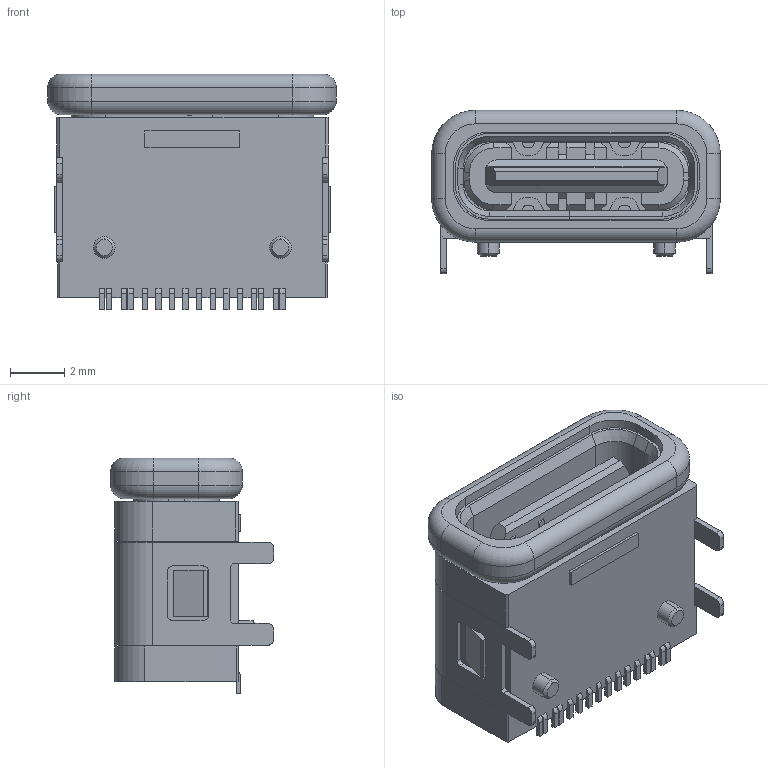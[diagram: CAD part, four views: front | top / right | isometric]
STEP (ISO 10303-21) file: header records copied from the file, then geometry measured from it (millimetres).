
FILE_DESCRIPTION (( 'STEP AP214' ), '1' );
FILE_NAME ('698B116W163-601.STEP', '2021-01-15T13:41:08', ( '' ), ( '' ), 'SwSTEP 2.0', 'SolidWorks 2020', '' );
FILE_SCHEMA (( 'AUTOMOTIVE_DESIGN' ));
Length unit declared in the file: millimetre
Products named in the file (5): Shell1 698B116WX63-601; 698B116WX63-601 (Seal); Shell2 698B116WX63-601; 698B116W163-601; Insulator 698B116WX63-601
Assembly tree (4 placements, depth 2):
  698B116W163-601
    Insulator 698B116WX63-601
    Shell1 698B116WX63-601
    Shell2 698B116WX63-601
    698B116WX63-601 (Seal)
Bounding box: 10.64 x 6.01 x 8.7 mm (x, y, z)
Volume: 284 mm3; surface area: 999.6 mm2
Topology: 4 solids, 4 shells, 633 faces, 1787 edges, 1162 vertices
Faces by surface type: plane 449, cylinder 164, cone 12, torus 8
Entity records: 21702 total; most frequent: CARTESIAN_POINT 3820, ORIENTED_EDGE 3574, DIRECTION 3370, EDGE_CURVE 1787, VECTOR 1410, LINE 1410, VERTEX_POINT 1162, AXIS2_PLACEMENT_3D 980
